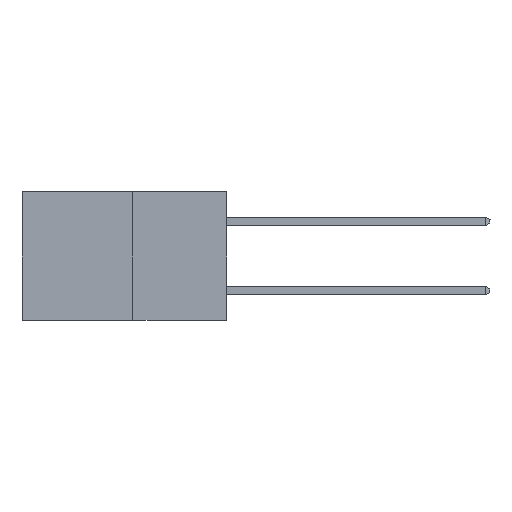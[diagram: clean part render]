
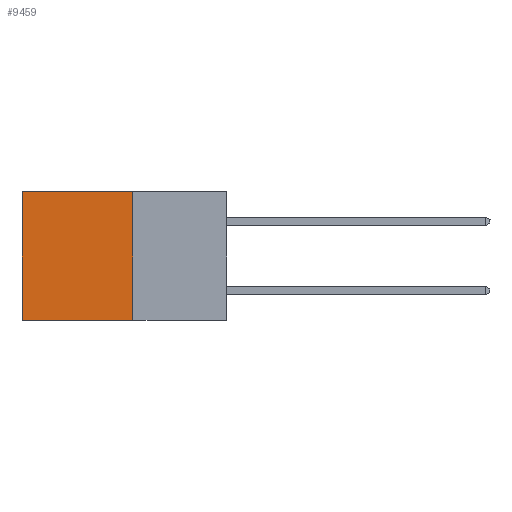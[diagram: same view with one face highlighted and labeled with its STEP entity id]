
A CAD part, left-side view. The second image highlights one B-rep face of the part: STEP entity #9459.
In plain terms, the highlighted planar face has unit normal (-1, 0, 0).
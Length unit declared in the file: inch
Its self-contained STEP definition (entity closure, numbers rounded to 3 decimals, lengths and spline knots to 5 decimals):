
#542 = VERTEX_POINT ( 'NONE', #17703 ) ;
#1009 = CARTESIAN_POINT ( 'NONE',  ( 0.277, 0.27, 0. ) ) ;
#2692 = LINE ( 'NONE', #19965, #22672 ) ;
#2825 = EDGE_CURVE ( 'NONE', #8559, #20235, #22439, .T. ) ;
#3853 = AXIS2_PLACEMENT_3D ( 'NONE', #5803, #13700, #31885 ) ;
#5803 = CARTESIAN_POINT ( 'NONE',  ( 0.277, 0.27, -0.37 ) ) ;
#6652 = DIRECTION ( 'NONE',  ( 0., 1., 0. ) ) ;
#6833 = ORIENTED_EDGE ( 'NONE', *, *, #21140, .F. ) ;
#6985 = DIRECTION ( 'NONE',  ( 0., 0., -1. ) ) ;
#7274 = CARTESIAN_POINT ( 'NONE',  ( 0.277, 0.27, 0. ) ) ;
#8068 = CARTESIAN_POINT ( 'NONE',  ( 0.277, 0.59, -0.37 ) ) ;
#8456 = LINE ( 'NONE', #1009, #21481 ) ;
#8559 = VERTEX_POINT ( 'NONE', #12379 ) ;
#9441 = VECTOR ( 'NONE', #6652, 39.37008 ) ;
#9459 = ADVANCED_FACE ( 'NONE', ( #25467 ), #24036, .F. ) ;
#12136 = EDGE_CURVE ( 'NONE', #542, #20235, #28157, .T. ) ;
#12379 = CARTESIAN_POINT ( 'NONE',  ( 0.277, 0.27, -0.37 ) ) ;
#12598 = VERTEX_POINT ( 'NONE', #7274 ) ;
#12723 = VECTOR ( 'NONE', #26425, 39.37008 ) ;
#13700 = DIRECTION ( 'NONE',  ( 1., 0., 0. ) ) ;
#13855 = ORIENTED_EDGE ( 'NONE', *, *, #20953, .T. ) ;
#17703 = CARTESIAN_POINT ( 'NONE',  ( 0.277, 0.59, 0. ) ) ;
#18190 = CARTESIAN_POINT ( 'NONE',  ( 0.277, 0.27, -0.37 ) ) ;
#18568 = CARTESIAN_POINT ( 'NONE',  ( 0.277, 0.59, -0.37 ) ) ;
#19965 = CARTESIAN_POINT ( 'NONE',  ( 0.277, 0.27, -0.37 ) ) ;
#20235 = VERTEX_POINT ( 'NONE', #8068 ) ;
#20953 = EDGE_CURVE ( 'NONE', #12598, #542, #8456, .T. ) ;
#21140 = EDGE_CURVE ( 'NONE', #12598, #8559, #2692, .T. ) ;
#21481 = VECTOR ( 'NONE', #21912, 39.37008 ) ;
#21816 = ORIENTED_EDGE ( 'NONE', *, *, #12136, .T. ) ;
#21912 = DIRECTION ( 'NONE',  ( 0., 1., 0. ) ) ;
#22439 = LINE ( 'NONE', #18190, #9441 ) ;
#22672 = VECTOR ( 'NONE', #6985, 39.37008 ) ;
#24036 = PLANE ( 'NONE',  #3853 ) ;
#25467 = FACE_OUTER_BOUND ( 'NONE', #27680, .T. ) ;
#26425 = DIRECTION ( 'NONE',  ( 0., 0., -1. ) ) ;
#27680 = EDGE_LOOP ( 'NONE', ( #21816, #31525, #6833, #13855 ) ) ;
#28157 = LINE ( 'NONE', #18568, #12723 ) ;
#31525 = ORIENTED_EDGE ( 'NONE', *, *, #2825, .F. ) ;
#31885 = DIRECTION ( 'NONE',  ( 0., 0., -1. ) ) ;
